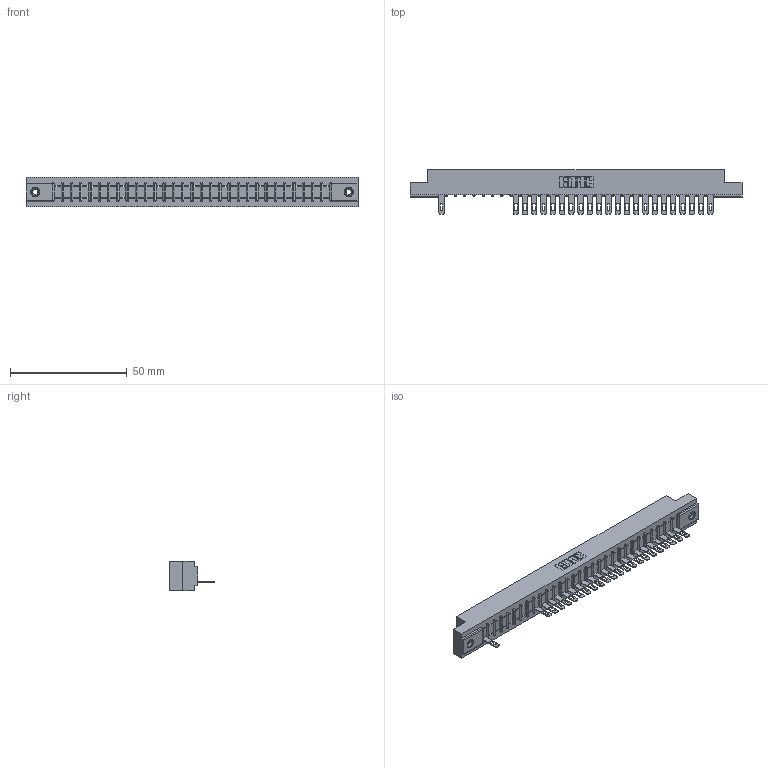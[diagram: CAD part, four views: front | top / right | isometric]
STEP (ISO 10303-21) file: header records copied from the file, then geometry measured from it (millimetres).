
FILE_DESCRIPTION (( 'STEP AP203' ), '1' );
FILE_NAME ('357-030-505-108.STEP', '2018-08-09T08:28:27', ( '' ), ( '' ), 'SwSTEP 2.0', 'SolidWorks 2016', '' );
FILE_SCHEMA (( 'CONFIG_CONTROL_DESIGN' ));
Length unit declared in the file: inch
Products named in the file (4): 345-250-001_345-250-003-102; 357-030-505-108; 307 Part_.156 Dia Mounting Holes; 307-290-001_505
Assembly tree (26 placements, depth 2):
  357-030-505-108
    307 Part_.156 Dia Mounting Holes
    307-290-001_505  x23
    345-250-001_345-250-003-102  x2
Bounding box: 141.88 x 19.18 x 12.7 mm (x, y, z)
Volume: 14584.1 mm3; surface area: 14850.5 mm2
Topology: 26 solids, 26 shells, 1637 faces, 4633 edges, 2966 vertices
Faces by surface type: plane 1014, cylinder 545, sphere 62, cone 12, torus 4
Entity records: 28133 total; most frequent: CARTESIAN_POINT 4744, ORIENTED_EDGE 4730, DIRECTION 4625, EDGE_CURVE 2365, VECTOR 1807, LINE 1807, VERTEX_POINT 1528, AXIS2_PLACEMENT_3D 1409
